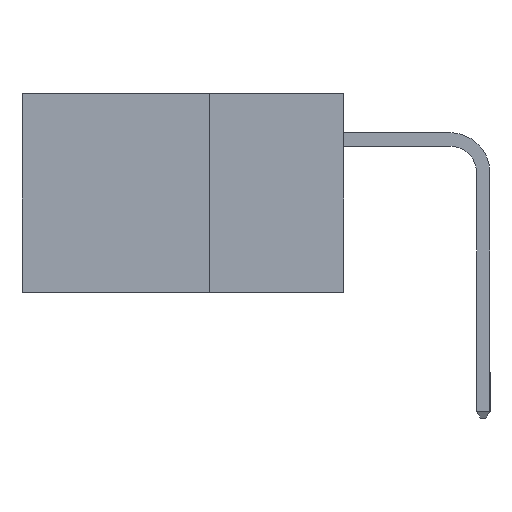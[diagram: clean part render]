
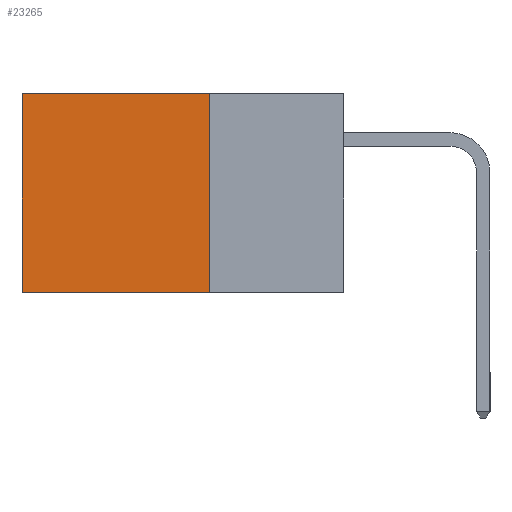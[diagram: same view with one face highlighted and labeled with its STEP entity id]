
A CAD part, left-side view. The second image highlights one B-rep face of the part: STEP entity #23265.
In plain terms, the highlighted planar face has unit normal (-1, 0, 0).
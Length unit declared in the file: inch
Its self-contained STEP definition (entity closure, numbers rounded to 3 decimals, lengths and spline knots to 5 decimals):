
#106 = CARTESIAN_POINT ( 'NONE',  ( 0.298, 0.6, 0. ) ) ;
#526 = VERTEX_POINT ( 'NONE', #23935 ) ;
#1936 = DIRECTION ( 'NONE',  ( 1., 0., 0. ) ) ;
#3053 = DIRECTION ( 'NONE',  ( 0., 1., 0. ) ) ;
#4382 = EDGE_CURVE ( 'NONE', #13778, #526, #9460, .T. ) ;
#5420 = ORIENTED_EDGE ( 'NONE', *, *, #10038, .F. ) ;
#6160 = FACE_OUTER_BOUND ( 'NONE', #6403, .T. ) ;
#6358 = CARTESIAN_POINT ( 'NONE',  ( 0.298, 0.25, 0. ) ) ;
#6403 = EDGE_LOOP ( 'NONE', ( #21488, #5420, #26200, #18174 ) ) ;
#8261 = VECTOR ( 'NONE', #3053, 39.37008 ) ;
#9460 = LINE ( 'NONE', #6358, #16595 ) ;
#10038 = EDGE_CURVE ( 'NONE', #526, #28971, #19117, .T. ) ;
#10394 = CARTESIAN_POINT ( 'NONE',  ( 0.298, 0.6, 0. ) ) ;
#11676 = DIRECTION ( 'NONE',  ( 0., 0., -1. ) ) ;
#13422 = VECTOR ( 'NONE', #18560, 39.37008 ) ;
#13778 = VERTEX_POINT ( 'NONE', #28708 ) ;
#13862 = CARTESIAN_POINT ( 'NONE',  ( 0.298, 0.25, 0. ) ) ;
#14953 = DIRECTION ( 'NONE',  ( 0., 1., 0. ) ) ;
#15309 = VECTOR ( 'NONE', #14953, 39.37008 ) ;
#16595 = VECTOR ( 'NONE', #27847, 39.37008 ) ;
#18174 = ORIENTED_EDGE ( 'NONE', *, *, #26556, .T. ) ;
#18430 = PLANE ( 'NONE',  #28189 ) ;
#18560 = DIRECTION ( 'NONE',  ( 0., 0., -1. ) ) ;
#19117 = LINE ( 'NONE', #28911, #8261 ) ;
#20567 = VERTEX_POINT ( 'NONE', #10394 ) ;
#20644 = LINE ( 'NONE', #106, #13422 ) ;
#21488 = ORIENTED_EDGE ( 'NONE', *, *, #23135, .T. ) ;
#23135 = EDGE_CURVE ( 'NONE', #20567, #28971, #20644, .T. ) ;
#23265 = ADVANCED_FACE ( 'NONE', ( #6160 ), #18430, .F. ) ;
#23935 = CARTESIAN_POINT ( 'NONE',  ( 0.298, 0.25, -0.37 ) ) ;
#24138 = CARTESIAN_POINT ( 'NONE',  ( 0.298, 0.25, 0. ) ) ;
#26200 = ORIENTED_EDGE ( 'NONE', *, *, #4382, .F. ) ;
#26556 = EDGE_CURVE ( 'NONE', #13778, #20567, #27338, .T. ) ;
#26907 = CARTESIAN_POINT ( 'NONE',  ( 0.298, 0.6, -0.37 ) ) ;
#27338 = LINE ( 'NONE', #24138, #15309 ) ;
#27847 = DIRECTION ( 'NONE',  ( 0., 0., -1. ) ) ;
#28189 = AXIS2_PLACEMENT_3D ( 'NONE', #13862, #1936, #11676 ) ;
#28708 = CARTESIAN_POINT ( 'NONE',  ( 0.298, 0.25, 0. ) ) ;
#28911 = CARTESIAN_POINT ( 'NONE',  ( 0.298, 0.25, -0.37 ) ) ;
#28971 = VERTEX_POINT ( 'NONE', #26907 ) ;
